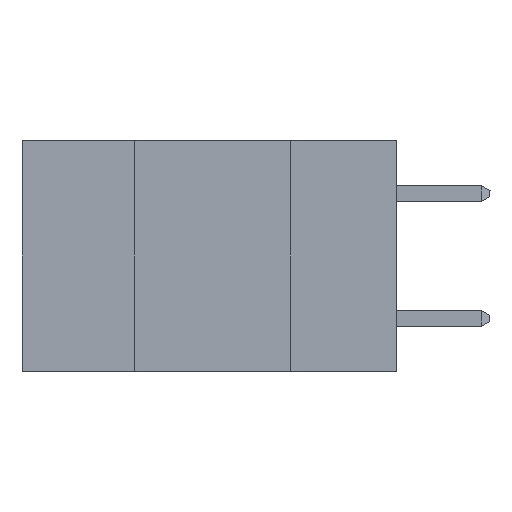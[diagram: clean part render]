
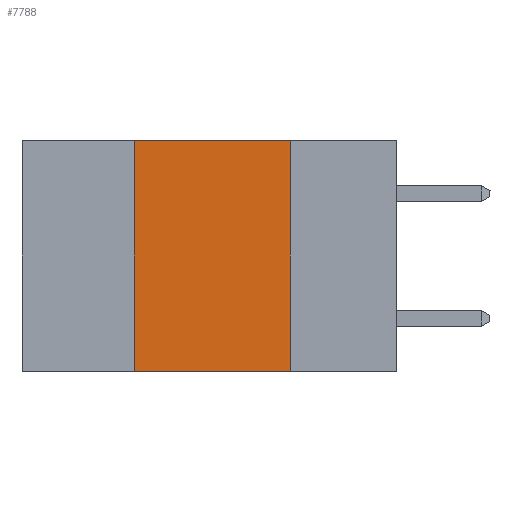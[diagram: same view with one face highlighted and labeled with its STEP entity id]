
A CAD part, left-side view. The second image highlights one B-rep face of the part: STEP entity #7788.
In plain terms, the highlighted planar face has unit normal (-1, 0, 0).
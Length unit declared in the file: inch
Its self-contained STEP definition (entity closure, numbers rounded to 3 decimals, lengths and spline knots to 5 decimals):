
#176 = CARTESIAN_POINT ( 'NONE',  ( 0., 0.42, -0.37 ) ) ;
#290 = CARTESIAN_POINT ( 'NONE',  ( 0., 0.6, 0. ) ) ;
#538 = DIRECTION ( 'NONE',  ( 1., 0., 0. ) ) ;
#1018 = DIRECTION ( 'NONE',  ( 0., 0., -1. ) ) ;
#2355 = EDGE_CURVE ( 'NONE', #9872, #2621, #14315, .T. ) ;
#2552 = DIRECTION ( 'NONE',  ( 0., 0., 1. ) ) ;
#2621 = VERTEX_POINT ( 'NONE', #11253 ) ;
#3947 = VECTOR ( 'NONE', #9758, 39.37008 ) ;
#5348 = VECTOR ( 'NONE', #1018, 39.37008 ) ;
#5429 = ORIENTED_EDGE ( 'NONE', *, *, #13662, .T. ) ;
#5797 = ORIENTED_EDGE ( 'NONE', *, *, #2355, .F. ) ;
#5888 = LINE ( 'NONE', #8461, #11727 ) ;
#6225 = CARTESIAN_POINT ( 'NONE',  ( 0., 0.6, 0. ) ) ;
#6351 = ORIENTED_EDGE ( 'NONE', *, *, #10499, .F. ) ;
#6383 = CARTESIAN_POINT ( 'NONE',  ( 0., 0.17, -0.37 ) ) ;
#7624 = FACE_OUTER_BOUND ( 'NONE', #7828, .T. ) ;
#7788 = ADVANCED_FACE ( 'NONE', ( #7624 ), #9871, .F. ) ;
#7828 = EDGE_LOOP ( 'NONE', ( #6351, #5797, #10548, #5429 ) ) ;
#8063 = VECTOR ( 'NONE', #9191, 39.37008 ) ;
#8439 = LINE ( 'NONE', #15154, #5348 ) ;
#8461 = CARTESIAN_POINT ( 'NONE',  ( 0., 0.42, 0. ) ) ;
#8960 = VERTEX_POINT ( 'NONE', #6383 ) ;
#9191 = DIRECTION ( 'NONE',  ( 0., -1., 0. ) ) ;
#9758 = DIRECTION ( 'NONE',  ( 0., -1., 0. ) ) ;
#9871 = PLANE ( 'NONE',  #13233 ) ;
#9872 = VERTEX_POINT ( 'NONE', #15029 ) ;
#10499 = EDGE_CURVE ( 'NONE', #2621, #8960, #8439, .T. ) ;
#10548 = ORIENTED_EDGE ( 'NONE', *, *, #10696, .F. ) ;
#10696 = EDGE_CURVE ( 'NONE', #11391, #9872, #5888, .T. ) ;
#10935 = DIRECTION ( 'NONE',  ( 0., 0., -1. ) ) ;
#11253 = CARTESIAN_POINT ( 'NONE',  ( 0., 0.17, 0. ) ) ;
#11391 = VERTEX_POINT ( 'NONE', #176 ) ;
#11727 = VECTOR ( 'NONE', #2552, 39.37008 ) ;
#12082 = CARTESIAN_POINT ( 'NONE',  ( 0., 0.6, -0.37 ) ) ;
#12927 = LINE ( 'NONE', #12082, #3947 ) ;
#13233 = AXIS2_PLACEMENT_3D ( 'NONE', #290, #538, #10935 ) ;
#13662 = EDGE_CURVE ( 'NONE', #11391, #8960, #12927, .T. ) ;
#14315 = LINE ( 'NONE', #6225, #8063 ) ;
#15029 = CARTESIAN_POINT ( 'NONE',  ( 0., 0.42, 0. ) ) ;
#15154 = CARTESIAN_POINT ( 'NONE',  ( 0., 0.17, 0. ) ) ;
